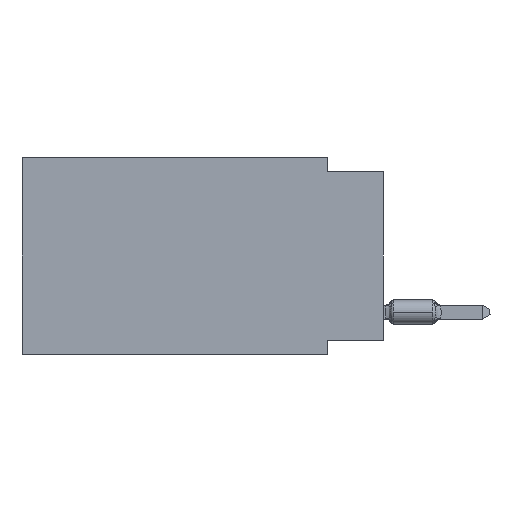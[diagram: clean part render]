
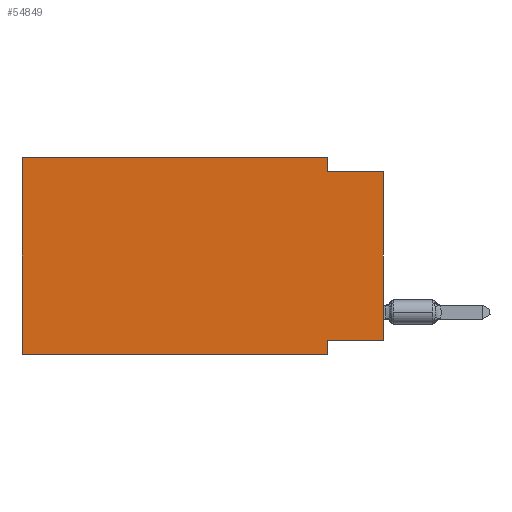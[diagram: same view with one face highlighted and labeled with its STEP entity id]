
A CAD part, left-side view. The second image highlights one B-rep face of the part: STEP entity #54849.
In plain terms, the highlighted planar face has unit normal (-1, 0, 0).
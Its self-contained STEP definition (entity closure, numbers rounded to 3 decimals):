
#2130 = DIRECTION ( 'NONE',  ( 0., -1., 0. ) ) ;
#2434 = VECTOR ( 'NONE', #25432, 1000. ) ;
#3091 = DIRECTION ( 'NONE',  ( 0., 1., 0. ) ) ;
#3203 = EDGE_CURVE ( 'NONE', #42196, #4938, #55387, .T. ) ;
#4194 = DIRECTION ( 'NONE',  ( 0., 0., 1. ) ) ;
#4938 = VERTEX_POINT ( 'NONE', #58425 ) ;
#5426 = CARTESIAN_POINT ( 'NONE',  ( 0., 0., -0.635 ) ) ;
#5734 = VERTEX_POINT ( 'NONE', #33881 ) ;
#5814 = FACE_OUTER_BOUND ( 'NONE', #55653, .T. ) ;
#7009 = ORIENTED_EDGE ( 'NONE', *, *, #38958, .F. ) ;
#7322 = CARTESIAN_POINT ( 'NONE',  ( 0., 16.383, 0. ) ) ;
#9578 = LINE ( 'NONE', #32450, #54911 ) ;
#10829 = DIRECTION ( 'NONE',  ( 0., 0., -1. ) ) ;
#11463 = CARTESIAN_POINT ( 'NONE',  ( 0., 0., -0.635 ) ) ;
#15734 = CARTESIAN_POINT ( 'NONE',  ( 0., 2.54, 0. ) ) ;
#16317 = CARTESIAN_POINT ( 'NONE',  ( 0., 2.54, -8.255 ) ) ;
#17404 = ORIENTED_EDGE ( 'NONE', *, *, #18867, .F. ) ;
#17511 = ORIENTED_EDGE ( 'NONE', *, *, #56151, .F. ) ;
#17886 = DIRECTION ( 'NONE',  ( 0., 0., -1. ) ) ;
#17919 = ORIENTED_EDGE ( 'NONE', *, *, #27463, .F. ) ;
#18867 = EDGE_CURVE ( 'NONE', #4938, #36415, #24056, .T. ) ;
#19619 = VERTEX_POINT ( 'NONE', #5426 ) ;
#20008 = VERTEX_POINT ( 'NONE', #16317 ) ;
#20820 = LINE ( 'NONE', #33901, #45087 ) ;
#21347 = CARTESIAN_POINT ( 'NONE',  ( 0., 16.383, -8.89 ) ) ;
#21497 = CARTESIAN_POINT ( 'NONE',  ( 0., 0., -8.255 ) ) ;
#21865 = EDGE_CURVE ( 'NONE', #20008, #49313, #9578, .T. ) ;
#23085 = CARTESIAN_POINT ( 'NONE',  ( 0., 16.383, 0. ) ) ;
#24056 = LINE ( 'NONE', #15734, #41280 ) ;
#24432 = CARTESIAN_POINT ( 'NONE',  ( 0., 2.54, -8.89 ) ) ;
#25432 = DIRECTION ( 'NONE',  ( 0., -1., 0. ) ) ;
#26802 = LINE ( 'NONE', #49361, #26998 ) ;
#26998 = VECTOR ( 'NONE', #4194, 1000. ) ;
#27463 = EDGE_CURVE ( 'NONE', #36415, #19619, #34341, .T. ) ;
#28822 = DIRECTION ( 'NONE',  ( 0., 0., -1. ) ) ;
#32450 = CARTESIAN_POINT ( 'NONE',  ( 0., 2.54, -8.89 ) ) ;
#32590 = LINE ( 'NONE', #23085, #54112 ) ;
#33881 = CARTESIAN_POINT ( 'NONE',  ( 0., 0., -8.255 ) ) ;
#33901 = CARTESIAN_POINT ( 'NONE',  ( 0., 16.383, -8.89 ) ) ;
#34341 = LINE ( 'NONE', #11463, #2434 ) ;
#36415 = VERTEX_POINT ( 'NONE', #42480 ) ;
#37408 = AXIS2_PLACEMENT_3D ( 'NONE', #50383, #41758, #10829 ) ;
#38113 = ORIENTED_EDGE ( 'NONE', *, *, #50322, .T. ) ;
#38472 = LINE ( 'NONE', #21497, #55441 ) ;
#38738 = ORIENTED_EDGE ( 'NONE', *, *, #3203, .F. ) ;
#38958 = EDGE_CURVE ( 'NONE', #57098, #42196, #32590, .T. ) ;
#41206 = DIRECTION ( 'NONE',  ( 0., 0., 1. ) ) ;
#41280 = VECTOR ( 'NONE', #28822, 1000. ) ;
#41420 = CARTESIAN_POINT ( 'NONE',  ( 0., 16.383, 0. ) ) ;
#41758 = DIRECTION ( 'NONE',  ( 1., 0., 0. ) ) ;
#42196 = VERTEX_POINT ( 'NONE', #7322 ) ;
#42480 = CARTESIAN_POINT ( 'NONE',  ( 0., 2.54, -0.635 ) ) ;
#45087 = VECTOR ( 'NONE', #2130, 1000. ) ;
#45594 = DIRECTION ( 'NONE',  ( 0., -1., 0. ) ) ;
#47539 = ORIENTED_EDGE ( 'NONE', *, *, #52924, .T. ) ;
#49313 = VERTEX_POINT ( 'NONE', #24432 ) ;
#49361 = CARTESIAN_POINT ( 'NONE',  ( 0., 0., 0. ) ) ;
#50322 = EDGE_CURVE ( 'NONE', #5734, #19619, #26802, .T. ) ;
#50383 = CARTESIAN_POINT ( 'NONE',  ( 0., 16.383, 0. ) ) ;
#52924 = EDGE_CURVE ( 'NONE', #57098, #49313, #20820, .T. ) ;
#53358 = ORIENTED_EDGE ( 'NONE', *, *, #21865, .F. ) ;
#53638 = VECTOR ( 'NONE', #45594, 1000. ) ;
#54112 = VECTOR ( 'NONE', #41206, 1000. ) ;
#54849 = ADVANCED_FACE ( 'NONE', ( #5814 ), #55416, .F. ) ;
#54911 = VECTOR ( 'NONE', #17886, 1000. ) ;
#55387 = LINE ( 'NONE', #41420, #53638 ) ;
#55416 = PLANE ( 'NONE',  #37408 ) ;
#55441 = VECTOR ( 'NONE', #3091, 1000. ) ;
#55653 = EDGE_LOOP ( 'NONE', ( #38113, #17919, #17404, #38738, #7009, #47539, #53358, #17511 ) ) ;
#56151 = EDGE_CURVE ( 'NONE', #5734, #20008, #38472, .T. ) ;
#57098 = VERTEX_POINT ( 'NONE', #21347 ) ;
#58425 = CARTESIAN_POINT ( 'NONE',  ( 0., 2.54, 0. ) ) ;
